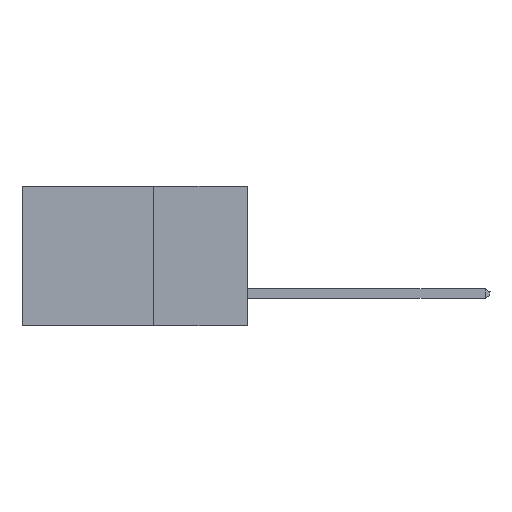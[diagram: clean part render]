
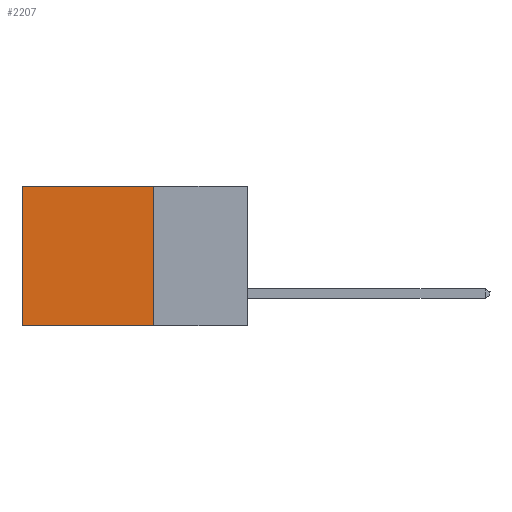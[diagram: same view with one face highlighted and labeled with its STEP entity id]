
A CAD part, left-side view. The second image highlights one B-rep face of the part: STEP entity #2207.
In plain terms, the highlighted planar face has unit normal (-1, 0, 0).
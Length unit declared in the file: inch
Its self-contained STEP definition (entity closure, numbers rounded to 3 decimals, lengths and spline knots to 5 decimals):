
#315 = AXIS2_PLACEMENT_3D ( 'NONE', #2060, #15715, #9518 ) ;
#783 = CARTESIAN_POINT ( 'NONE',  ( 0.2615, 0.6, 0. ) ) ;
#856 = LINE ( 'NONE', #2409, #4070 ) ;
#1411 = CARTESIAN_POINT ( 'NONE',  ( 0.2615, 0.25, -0.37 ) ) ;
#2060 = CARTESIAN_POINT ( 'NONE',  ( 0.2615, 0.25, -0.37 ) ) ;
#2207 = ADVANCED_FACE ( 'NONE', ( #4918 ), #7023, .F. ) ;
#2409 = CARTESIAN_POINT ( 'NONE',  ( 0.2615, 0.6, -0.37 ) ) ;
#2533 = CARTESIAN_POINT ( 'NONE',  ( 0.2615, 0.25, 0. ) ) ;
#2855 = VERTEX_POINT ( 'NONE', #10378 ) ;
#3817 = CARTESIAN_POINT ( 'NONE',  ( 0.2615, 0.6, -0.37 ) ) ;
#3942 = DIRECTION ( 'NONE',  ( 0., 0., -1. ) ) ;
#4070 = VECTOR ( 'NONE', #15822, 39.37008 ) ;
#4110 = EDGE_CURVE ( 'NONE', #5159, #12005, #13904, .T. ) ;
#4535 = VECTOR ( 'NONE', #5134, 39.37008 ) ;
#4918 = FACE_OUTER_BOUND ( 'NONE', #12707, .T. ) ;
#5134 = DIRECTION ( 'NONE',  ( 0., 1., 0. ) ) ;
#5159 = VERTEX_POINT ( 'NONE', #14098 ) ;
#6119 = DIRECTION ( 'NONE',  ( 0., 1., 0. ) ) ;
#7023 = PLANE ( 'NONE',  #315 ) ;
#7586 = LINE ( 'NONE', #1411, #13265 ) ;
#7843 = VECTOR ( 'NONE', #6119, 39.37008 ) ;
#7846 = ORIENTED_EDGE ( 'NONE', *, *, #14915, .F. ) ;
#7860 = EDGE_CURVE ( 'NONE', #12005, #8722, #856, .T. ) ;
#8096 = ORIENTED_EDGE ( 'NONE', *, *, #4110, .T. ) ;
#8593 = CARTESIAN_POINT ( 'NONE',  ( 0.2615, 0.25, -0.37 ) ) ;
#8722 = VERTEX_POINT ( 'NONE', #3817 ) ;
#9518 = DIRECTION ( 'NONE',  ( 0., 0., -1. ) ) ;
#10378 = CARTESIAN_POINT ( 'NONE',  ( 0.2615, 0.25, -0.37 ) ) ;
#12005 = VERTEX_POINT ( 'NONE', #783 ) ;
#12707 = EDGE_LOOP ( 'NONE', ( #15806, #13132, #7846, #8096 ) ) ;
#13132 = ORIENTED_EDGE ( 'NONE', *, *, #15527, .F. ) ;
#13260 = LINE ( 'NONE', #8593, #7843 ) ;
#13265 = VECTOR ( 'NONE', #3942, 39.37008 ) ;
#13904 = LINE ( 'NONE', #2533, #4535 ) ;
#14098 = CARTESIAN_POINT ( 'NONE',  ( 0.2615, 0.25, 0. ) ) ;
#14915 = EDGE_CURVE ( 'NONE', #5159, #2855, #7586, .T. ) ;
#15527 = EDGE_CURVE ( 'NONE', #2855, #8722, #13260, .T. ) ;
#15715 = DIRECTION ( 'NONE',  ( 1., 0., 0. ) ) ;
#15806 = ORIENTED_EDGE ( 'NONE', *, *, #7860, .T. ) ;
#15822 = DIRECTION ( 'NONE',  ( 0., 0., -1. ) ) ;
